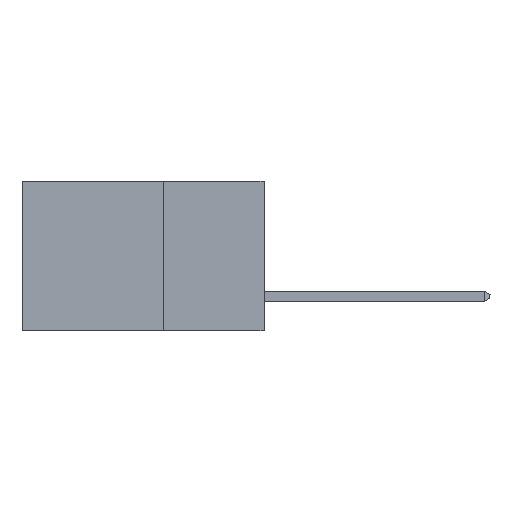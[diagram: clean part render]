
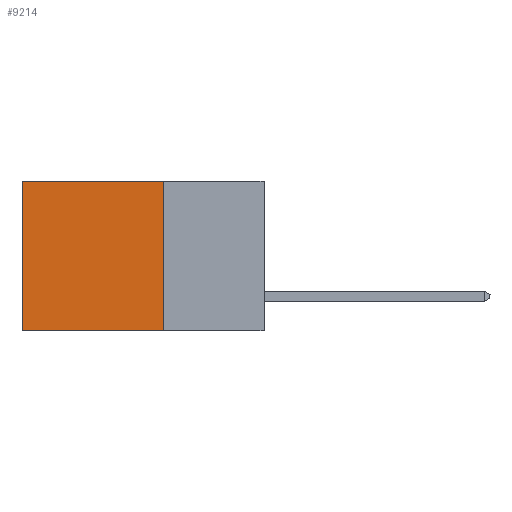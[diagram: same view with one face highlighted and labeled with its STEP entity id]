
A CAD part, left-side view. The second image highlights one B-rep face of the part: STEP entity #9214.
In plain terms, the highlighted planar face has unit normal (-1, 0, 0).
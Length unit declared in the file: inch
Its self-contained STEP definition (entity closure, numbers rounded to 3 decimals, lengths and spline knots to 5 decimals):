
#123 = CARTESIAN_POINT ( 'NONE',  ( 0.298, 0.25, -0.37 ) ) ;
#368 = CARTESIAN_POINT ( 'NONE',  ( 0.298, 0.25, 0. ) ) ;
#410 = CARTESIAN_POINT ( 'NONE',  ( 0.298, 0.6, 0. ) ) ;
#1177 = CARTESIAN_POINT ( 'NONE',  ( 0.298, 0.25, 0. ) ) ;
#1587 = LINE ( 'NONE', #8409, #3362 ) ;
#1775 = VECTOR ( 'NONE', #8280, 39.37008 ) ;
#1899 = CARTESIAN_POINT ( 'NONE',  ( 0.298, 0.25, 0. ) ) ;
#2702 = DIRECTION ( 'NONE',  ( 0., 1., 0. ) ) ;
#2823 = FACE_OUTER_BOUND ( 'NONE', #5033, .T. ) ;
#3278 = VERTEX_POINT ( 'NONE', #368 ) ;
#3362 = VECTOR ( 'NONE', #2702, 39.37008 ) ;
#4035 = ORIENTED_EDGE ( 'NONE', *, *, #9517, .T. ) ;
#4464 = LINE ( 'NONE', #1899, #5889 ) ;
#5033 = EDGE_LOOP ( 'NONE', ( #12087, #12044, #5247, #4035 ) ) ;
#5247 = ORIENTED_EDGE ( 'NONE', *, *, #7925, .F. ) ;
#5375 = CARTESIAN_POINT ( 'NONE',  ( 0.298, 0.6, -0.37 ) ) ;
#5889 = VECTOR ( 'NONE', #7523, 39.37008 ) ;
#6001 = VERTEX_POINT ( 'NONE', #123 ) ;
#7523 = DIRECTION ( 'NONE',  ( 0., 0., -1. ) ) ;
#7593 = PLANE ( 'NONE',  #11737 ) ;
#7748 = VERTEX_POINT ( 'NONE', #5375 ) ;
#7925 = EDGE_CURVE ( 'NONE', #3278, #6001, #4464, .T. ) ;
#7950 = VECTOR ( 'NONE', #10184, 39.37008 ) ;
#8224 = CARTESIAN_POINT ( 'NONE',  ( 0.298, 0.6, 0. ) ) ;
#8280 = DIRECTION ( 'NONE',  ( 0., 0., -1. ) ) ;
#8409 = CARTESIAN_POINT ( 'NONE',  ( 0.298, 0.25, -0.37 ) ) ;
#9214 = ADVANCED_FACE ( 'NONE', ( #2823 ), #7593, .F. ) ;
#9340 = EDGE_CURVE ( 'NONE', #11308, #7748, #11662, .T. ) ;
#9517 = EDGE_CURVE ( 'NONE', #3278, #11308, #14160, .T. ) ;
#9828 = DIRECTION ( 'NONE',  ( 0., 0., -1. ) ) ;
#9949 = EDGE_CURVE ( 'NONE', #6001, #7748, #1587, .T. ) ;
#10184 = DIRECTION ( 'NONE',  ( 0., 1., 0. ) ) ;
#10805 = CARTESIAN_POINT ( 'NONE',  ( 0.298, 0.25, 0. ) ) ;
#11308 = VERTEX_POINT ( 'NONE', #410 ) ;
#11662 = LINE ( 'NONE', #8224, #1775 ) ;
#11737 = AXIS2_PLACEMENT_3D ( 'NONE', #10805, #13157, #9828 ) ;
#12044 = ORIENTED_EDGE ( 'NONE', *, *, #9949, .F. ) ;
#12087 = ORIENTED_EDGE ( 'NONE', *, *, #9340, .T. ) ;
#13157 = DIRECTION ( 'NONE',  ( 1., 0., 0. ) ) ;
#14160 = LINE ( 'NONE', #1177, #7950 ) ;
